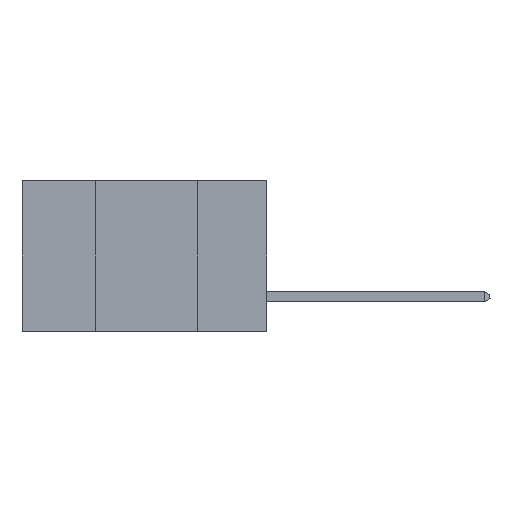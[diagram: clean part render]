
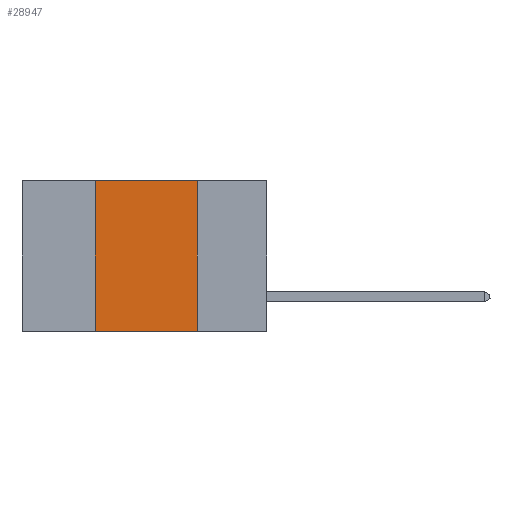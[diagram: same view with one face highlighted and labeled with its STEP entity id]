
A CAD part, left-side view. The second image highlights one B-rep face of the part: STEP entity #28947.
In plain terms, the highlighted planar face has unit normal (-1, 0, 0).
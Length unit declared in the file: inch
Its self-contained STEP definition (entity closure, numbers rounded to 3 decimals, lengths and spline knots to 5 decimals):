
#1356 = CARTESIAN_POINT ( 'NONE',  ( 0., 0.17, 0. ) ) ;
#2426 = EDGE_LOOP ( 'NONE', ( #30872, #33845, #31056, #33483 ) ) ;
#5480 = VECTOR ( 'NONE', #8464, 39.37008 ) ;
#6143 = PLANE ( 'NONE',  #45965 ) ;
#6746 = DIRECTION ( 'NONE',  ( 0., 0., -1. ) ) ;
#7623 = LINE ( 'NONE', #40329, #26587 ) ;
#8201 = VERTEX_POINT ( 'NONE', #1356 ) ;
#8464 = DIRECTION ( 'NONE',  ( 0., 0., 1. ) ) ;
#9135 = DIRECTION ( 'NONE',  ( 0., -1., 0. ) ) ;
#11212 = FACE_OUTER_BOUND ( 'NONE', #2426, .T. ) ;
#12139 = VECTOR ( 'NONE', #6746, 39.37008 ) ;
#13417 = DIRECTION ( 'NONE',  ( 0., 0., -1. ) ) ;
#15239 = VERTEX_POINT ( 'NONE', #28816 ) ;
#16448 = CARTESIAN_POINT ( 'NONE',  ( 0., 0.42, 0. ) ) ;
#17007 = VECTOR ( 'NONE', #9135, 39.37008 ) ;
#17504 = CARTESIAN_POINT ( 'NONE',  ( 0., 0.17, 0. ) ) ;
#18472 = EDGE_CURVE ( 'NONE', #15239, #38547, #7623, .T. ) ;
#20389 = CARTESIAN_POINT ( 'NONE',  ( 0., 0.6, 0. ) ) ;
#22248 = LINE ( 'NONE', #17504, #12139 ) ;
#26587 = VECTOR ( 'NONE', #44107, 39.37008 ) ;
#28816 = CARTESIAN_POINT ( 'NONE',  ( 0., 0.42, -0.37 ) ) ;
#28947 = ADVANCED_FACE ( 'NONE', ( #11212 ), #6143, .F. ) ;
#29295 = CARTESIAN_POINT ( 'NONE',  ( 0., 0.6, 0. ) ) ;
#29527 = CARTESIAN_POINT ( 'NONE',  ( 0., 0.17, -0.37 ) ) ;
#29770 = LINE ( 'NONE', #46205, #5480 ) ;
#30872 = ORIENTED_EDGE ( 'NONE', *, *, #31706, .F. ) ;
#31056 = ORIENTED_EDGE ( 'NONE', *, *, #37259, .F. ) ;
#31706 = EDGE_CURVE ( 'NONE', #8201, #38547, #22248, .T. ) ;
#32610 = DIRECTION ( 'NONE',  ( 1., 0., 0. ) ) ;
#33483 = ORIENTED_EDGE ( 'NONE', *, *, #18472, .T. ) ;
#33845 = ORIENTED_EDGE ( 'NONE', *, *, #46728, .F. ) ;
#37259 = EDGE_CURVE ( 'NONE', #15239, #48225, #29770, .T. ) ;
#38547 = VERTEX_POINT ( 'NONE', #29527 ) ;
#40329 = CARTESIAN_POINT ( 'NONE',  ( 0., 0.6, -0.37 ) ) ;
#43041 = LINE ( 'NONE', #20389, #17007 ) ;
#44107 = DIRECTION ( 'NONE',  ( 0., -1., 0. ) ) ;
#45965 = AXIS2_PLACEMENT_3D ( 'NONE', #29295, #32610, #13417 ) ;
#46205 = CARTESIAN_POINT ( 'NONE',  ( 0., 0.42, 0. ) ) ;
#46728 = EDGE_CURVE ( 'NONE', #48225, #8201, #43041, .T. ) ;
#48225 = VERTEX_POINT ( 'NONE', #16448 ) ;
